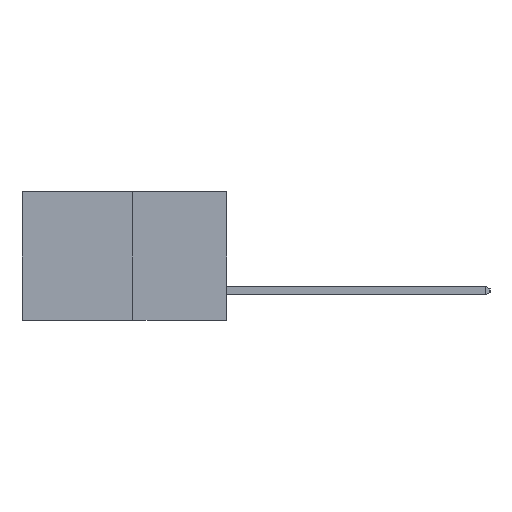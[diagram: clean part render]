
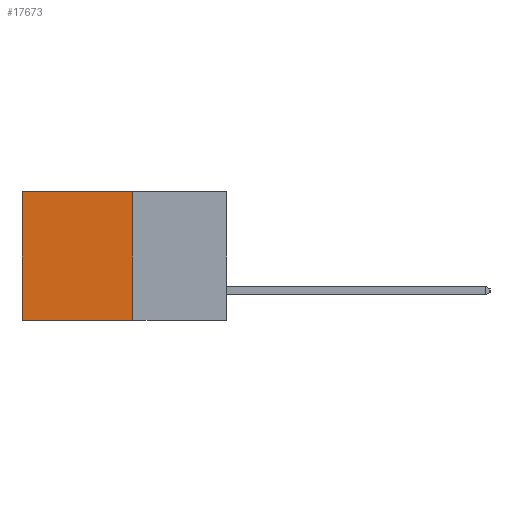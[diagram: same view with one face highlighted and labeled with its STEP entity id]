
A CAD part, left-side view. The second image highlights one B-rep face of the part: STEP entity #17673.
In plain terms, the highlighted planar face has unit normal (-1, 0, 0).
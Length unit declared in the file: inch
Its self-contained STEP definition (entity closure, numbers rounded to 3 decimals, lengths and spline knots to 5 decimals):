
#682 = CARTESIAN_POINT ( 'NONE',  ( 0.277, 0.59, 0. ) ) ;
#2099 = ORIENTED_EDGE ( 'NONE', *, *, #24067, .F. ) ;
#5290 = AXIS2_PLACEMENT_3D ( 'NONE', #14666, #5352, #21590 ) ;
#5352 = DIRECTION ( 'NONE',  ( 1., 0., 0. ) ) ;
#5371 = VECTOR ( 'NONE', #5561, 39.37008 ) ;
#5527 = CARTESIAN_POINT ( 'NONE',  ( 0.277, 0.27, 0. ) ) ;
#5561 = DIRECTION ( 'NONE',  ( 0., 0., -1. ) ) ;
#7616 = LINE ( 'NONE', #19486, #5371 ) ;
#9030 = EDGE_LOOP ( 'NONE', ( #27392, #2099, #21275, #26597 ) ) ;
#10266 = DIRECTION ( 'NONE',  ( 0., 1., 0. ) ) ;
#11095 = EDGE_CURVE ( 'NONE', #13631, #23720, #13837, .T. ) ;
#11593 = EDGE_CURVE ( 'NONE', #23720, #26228, #7616, .T. ) ;
#12364 = DIRECTION ( 'NONE',  ( 0., 0., -1. ) ) ;
#13474 = EDGE_CURVE ( 'NONE', #13631, #13589, #27804, .T. ) ;
#13589 = VERTEX_POINT ( 'NONE', #26312 ) ;
#13631 = VERTEX_POINT ( 'NONE', #22057 ) ;
#13837 = LINE ( 'NONE', #5527, #25273 ) ;
#14537 = VECTOR ( 'NONE', #25129, 39.37008 ) ;
#14666 = CARTESIAN_POINT ( 'NONE',  ( 0.277, 0.27, -0.37 ) ) ;
#17673 = ADVANCED_FACE ( 'NONE', ( #25473 ), #19304, .F. ) ;
#18924 = CARTESIAN_POINT ( 'NONE',  ( 0.277, 0.59, -0.37 ) ) ;
#19200 = CARTESIAN_POINT ( 'NONE',  ( 0.277, 0.27, -0.37 ) ) ;
#19304 = PLANE ( 'NONE',  #5290 ) ;
#19486 = CARTESIAN_POINT ( 'NONE',  ( 0.277, 0.59, -0.37 ) ) ;
#20566 = CARTESIAN_POINT ( 'NONE',  ( 0.277, 0.27, -0.37 ) ) ;
#21275 = ORIENTED_EDGE ( 'NONE', *, *, #13474, .F. ) ;
#21590 = DIRECTION ( 'NONE',  ( 0., 0., -1. ) ) ;
#21805 = VECTOR ( 'NONE', #12364, 39.37008 ) ;
#22057 = CARTESIAN_POINT ( 'NONE',  ( 0.277, 0.27, 0. ) ) ;
#23720 = VERTEX_POINT ( 'NONE', #682 ) ;
#24067 = EDGE_CURVE ( 'NONE', #13589, #26228, #26650, .T. ) ;
#25129 = DIRECTION ( 'NONE',  ( 0., 1., 0. ) ) ;
#25273 = VECTOR ( 'NONE', #10266, 39.37008 ) ;
#25473 = FACE_OUTER_BOUND ( 'NONE', #9030, .T. ) ;
#26228 = VERTEX_POINT ( 'NONE', #18924 ) ;
#26312 = CARTESIAN_POINT ( 'NONE',  ( 0.277, 0.27, -0.37 ) ) ;
#26597 = ORIENTED_EDGE ( 'NONE', *, *, #11095, .T. ) ;
#26650 = LINE ( 'NONE', #20566, #14537 ) ;
#27392 = ORIENTED_EDGE ( 'NONE', *, *, #11593, .T. ) ;
#27804 = LINE ( 'NONE', #19200, #21805 ) ;
